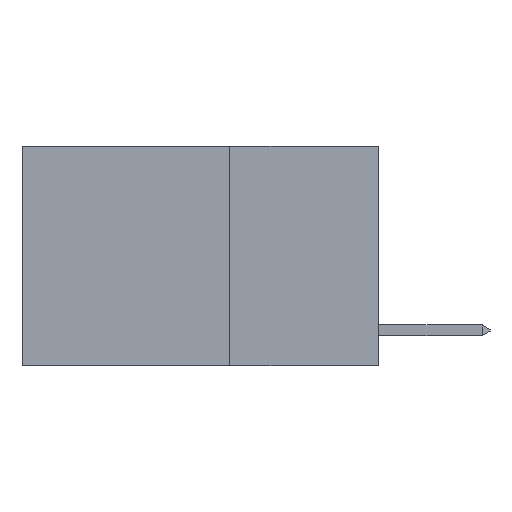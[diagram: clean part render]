
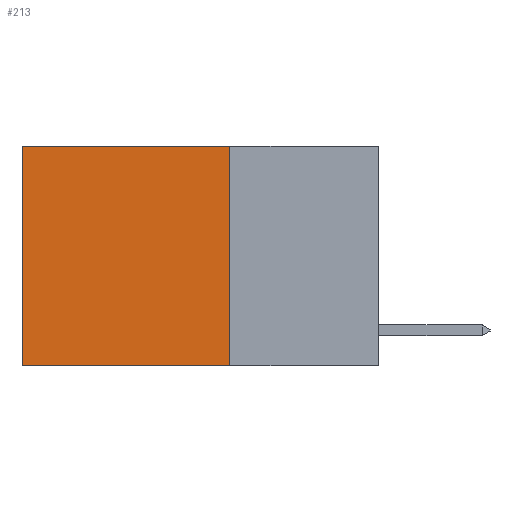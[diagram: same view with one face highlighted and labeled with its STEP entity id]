
A CAD part, left-side view. The second image highlights one B-rep face of the part: STEP entity #213.
In plain terms, the highlighted planar face has unit normal (-1, 0, 0).
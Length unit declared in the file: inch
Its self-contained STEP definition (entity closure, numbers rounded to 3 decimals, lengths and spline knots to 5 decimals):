
#104 = VERTEX_POINT ( 'NONE', #2336 ) ;
#113 = EDGE_LOOP ( 'NONE', ( #7987, #3054, #5222, #7458 ) ) ;
#213 = ADVANCED_FACE ( 'NONE', ( #5375 ), #533, .F. ) ;
#241 = VERTEX_POINT ( 'NONE', #3451 ) ;
#533 = PLANE ( 'NONE',  #3487 ) ;
#652 = CARTESIAN_POINT ( 'NONE',  ( 0.2625, 0.25, 0. ) ) ;
#681 = VECTOR ( 'NONE', #1915, 39.37008 ) ;
#1893 = VECTOR ( 'NONE', #6350, 39.37008 ) ;
#1915 = DIRECTION ( 'NONE',  ( 0., 1., 0. ) ) ;
#1994 = EDGE_CURVE ( 'NONE', #3825, #104, #9021, .T. ) ;
#2336 = CARTESIAN_POINT ( 'NONE',  ( 0.2625, 0.6, 0. ) ) ;
#2738 = CARTESIAN_POINT ( 'NONE',  ( 0.2625, 0.6, 0. ) ) ;
#2839 = DIRECTION ( 'NONE',  ( 0., 1., 0. ) ) ;
#2909 = CARTESIAN_POINT ( 'NONE',  ( 0.2625, 0.25, 0. ) ) ;
#3054 = ORIENTED_EDGE ( 'NONE', *, *, #8472, .F. ) ;
#3451 = CARTESIAN_POINT ( 'NONE',  ( 0.2625, 0.6, -0.37 ) ) ;
#3487 = AXIS2_PLACEMENT_3D ( 'NONE', #652, #6246, #7583 ) ;
#3505 = CARTESIAN_POINT ( 'NONE',  ( 0.2625, 0.25, 0. ) ) ;
#3517 = VECTOR ( 'NONE', #2839, 39.37008 ) ;
#3825 = VERTEX_POINT ( 'NONE', #6117 ) ;
#3890 = LINE ( 'NONE', #2738, #1893 ) ;
#4020 = EDGE_CURVE ( 'NONE', #3825, #8369, #4989, .T. ) ;
#4974 = DIRECTION ( 'NONE',  ( 0., 0., -1. ) ) ;
#4989 = LINE ( 'NONE', #3505, #6201 ) ;
#5222 = ORIENTED_EDGE ( 'NONE', *, *, #4020, .F. ) ;
#5375 = FACE_OUTER_BOUND ( 'NONE', #113, .T. ) ;
#6117 = CARTESIAN_POINT ( 'NONE',  ( 0.2625, 0.25, 0. ) ) ;
#6201 = VECTOR ( 'NONE', #4974, 39.37008 ) ;
#6246 = DIRECTION ( 'NONE',  ( 1., 0., 0. ) ) ;
#6251 = LINE ( 'NONE', #6963, #681 ) ;
#6350 = DIRECTION ( 'NONE',  ( 0., 0., -1. ) ) ;
#6963 = CARTESIAN_POINT ( 'NONE',  ( 0.2625, 0.25, -0.37 ) ) ;
#7458 = ORIENTED_EDGE ( 'NONE', *, *, #1994, .T. ) ;
#7524 = CARTESIAN_POINT ( 'NONE',  ( 0.2625, 0.25, -0.37 ) ) ;
#7583 = DIRECTION ( 'NONE',  ( 0., 0., -1. ) ) ;
#7987 = ORIENTED_EDGE ( 'NONE', *, *, #8518, .T. ) ;
#8369 = VERTEX_POINT ( 'NONE', #7524 ) ;
#8472 = EDGE_CURVE ( 'NONE', #8369, #241, #6251, .T. ) ;
#8518 = EDGE_CURVE ( 'NONE', #104, #241, #3890, .T. ) ;
#9021 = LINE ( 'NONE', #2909, #3517 ) ;
